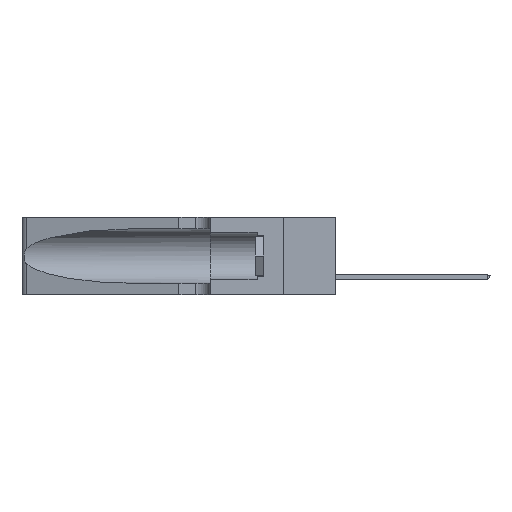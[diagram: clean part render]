
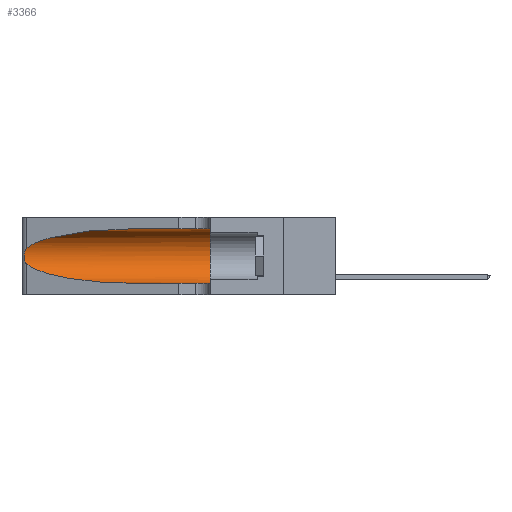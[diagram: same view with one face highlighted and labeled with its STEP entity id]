
A CAD part, left-side view. The second image highlights one B-rep face of the part: STEP entity #3366.
In plain terms, the highlighted cylindrical face has radius 3.308 mm (diameter 6.617 mm), a partial arc.
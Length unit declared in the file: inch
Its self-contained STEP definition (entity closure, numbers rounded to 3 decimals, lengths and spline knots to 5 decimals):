
#304 = CARTESIAN_POINT ( 'NONE',  ( 0.25487, 1.22718, 0.22369 ) ) ;
#501 = CARTESIAN_POINT ( 'NONE',  ( 0.1305, 0.72297, 0.05475 ) ) ;
#1171 = CARTESIAN_POINT ( 'NONE',  ( 0.26017, 1.23833, 0.17102 ) ) ;
#1795 = CARTESIAN_POINT ( 'NONE',  ( 0.1305, 0.35, 0.185 ) ) ;
#1953 = ORIENTED_EDGE ( 'NONE', *, *, #27291, .T. ) ;
#2363 = FACE_OUTER_BOUND ( 'NONE', #25673, .T. ) ;
#2447 = DIRECTION ( 'NONE',  ( 0., -1., 0. ) ) ;
#2669 = VERTEX_POINT ( 'NONE', #20504 ) ;
#2687 = CARTESIAN_POINT ( 'NONE',  ( 0.1305, 0.72297, 0.05475 ) ) ;
#2715 = VERTEX_POINT ( 'NONE', #11101 ) ;
#2776 = CARTESIAN_POINT ( 'NONE',  ( 0.25555, 1.22993, 0.14849 ) ) ;
#3366 = ADVANCED_FACE ( 'NONE', ( #2363 ), #10178, .F. ) ;
#3414 = CARTESIAN_POINT ( 'NONE',  ( 0.25639, 1.23186, 0.15144 ) ) ;
#3592 = LINE ( 'NONE', #9015, #15689 ) ;
#3740 = VERTEX_POINT ( 'NONE', #501 ) ;
#4025 = VERTEX_POINT ( 'NONE', #15299 ) ;
#4188 = EDGE_CURVE ( 'NONE', #17761, #4025, #16731, .T. ) ;
#4283 = CARTESIAN_POINT ( 'NONE',  ( 0.25487, 1.22718, 0.22369 ) ) ;
#4915 = ORIENTED_EDGE ( 'NONE', *, *, #13084, .T. ) ;
#5663 = EDGE_CURVE ( 'NONE', #22052, #2715, #14924, .T. ) ;
#6013 = ORIENTED_EDGE ( 'NONE', *, *, #15741, .T. ) ;
#6236 = DIRECTION ( 'NONE',  ( 0., 1., 0. ) ) ;
#6567 = CARTESIAN_POINT ( 'NONE',  ( 0.1305, 0.72297, 0.31525 ) ) ;
#7114 = CARTESIAN_POINT ( 'NONE',  ( 0.25487, 1.22718, 0.14631 ) ) ;
#9015 = CARTESIAN_POINT ( 'NONE',  ( 0.1305, 1.61858, 0.31525 ) ) ;
#9222 = CARTESIAN_POINT ( 'NONE',  ( 0.1305, 1.61858, 0.185 ) ) ;
#9841 = CARTESIAN_POINT ( 'NONE',  ( 0.25487, 1.22718, 0.22369 ) ) ;
#10178 = CYLINDRICAL_SURFACE ( 'NONE', #22697, 0.13025 ) ;
#11101 = CARTESIAN_POINT ( 'NONE',  ( 0.1305, 0.35, 0.05475 ) ) ;
#11452 =( BOUNDED_CURVE ( )  B_SPLINE_CURVE ( 3, ( #7114, #23000, #16283, #2687 ),
 .UNSPECIFIED., .F., .T. ) 
 B_SPLINE_CURVE_WITH_KNOTS ( ( 4, 4 ),
 ( 3.44316, 4.71239 ),
 .UNSPECIFIED. ) 
 CURVE ( )  GEOMETRIC_REPRESENTATION_ITEM ( )  RATIONAL_B_SPLINE_CURVE ( ( 1., 0.87, 0.87, 1. ) ) 
 REPRESENTATION_ITEM ( '' )  );
#11484 = ORIENTED_EDGE ( 'NONE', *, *, #4188, .T. ) ;
#11900 = CARTESIAN_POINT ( 'NONE',  ( 0.25854, 1.2359, 0.20912 ) ) ;
#12970 = ORIENTED_EDGE ( 'NONE', *, *, #5663, .F. ) ;
#13084 = EDGE_CURVE ( 'NONE', #2669, #17761, #27197, .T. ) ;
#14743 = CARTESIAN_POINT ( 'NONE',  ( 0.26075, 1.23896, 0.178 ) ) ;
#14924 = CIRCLE ( 'NONE', #28054, 0.13025 ) ;
#14928 = ORIENTED_EDGE ( 'NONE', *, *, #18840, .F. ) ;
#15299 = CARTESIAN_POINT ( 'NONE',  ( 0.25487, 1.22718, 0.14631 ) ) ;
#15689 = VECTOR ( 'NONE', #24651, 39.37008 ) ;
#15741 = EDGE_CURVE ( 'NONE', #4025, #3740, #11452, .T. ) ;
#15888 = DIRECTION ( 'NONE',  ( 0., 0., -1. ) ) ;
#16283 = CARTESIAN_POINT ( 'NONE',  ( 0.18966, 0.96281, 0.05475 ) ) ;
#16373 = CARTESIAN_POINT ( 'NONE',  ( 0.25789, 1.23486, 0.15765 ) ) ;
#16461 = CARTESIAN_POINT ( 'NONE',  ( 0.26018, 1.23835, 0.19895 ) ) ;
#16731 = B_SPLINE_CURVE_WITH_KNOTS ( 'NONE', 3,
 ( #304, #18436, #28000, #19046, #11900, #16461, #25520, #14743, #1171, #17009, #16373, #3414, #2776, #20946 ),
 .UNSPECIFIED., .F., .F.,
 ( 4, 2, 2, 2, 2, 2, 4 ),
 ( 0., 0.00027, 0.00053, 0.00107, 0.0016, 0.00187, 0.00214 ),
 .UNSPECIFIED. ) ;
#17009 = CARTESIAN_POINT ( 'NONE',  ( 0.25856, 1.23593, 0.16098 ) ) ;
#17761 = VERTEX_POINT ( 'NONE', #9841 ) ;
#18436 = CARTESIAN_POINT ( 'NONE',  ( 0.25555, 1.22994, 0.2215 ) ) ;
#18607 = CARTESIAN_POINT ( 'NONE',  ( 0.1305, 1.61858, 0.05475 ) ) ;
#18840 = EDGE_CURVE ( 'NONE', #2669, #22052, #3592, .T. ) ;
#19046 = CARTESIAN_POINT ( 'NONE',  ( 0.25787, 1.23484, 0.2124 ) ) ;
#20333 = CARTESIAN_POINT ( 'NONE',  ( 0.1305, 0.35, 0.31525 ) ) ;
#20504 = CARTESIAN_POINT ( 'NONE',  ( 0.1305, 0.72297, 0.31525 ) ) ;
#20729 = DIRECTION ( 'NONE',  ( 0., -1., 0. ) ) ;
#20922 = VECTOR ( 'NONE', #2447, 39.37008 ) ;
#20946 = CARTESIAN_POINT ( 'NONE',  ( 0.25487, 1.22718, 0.14631 ) ) ;
#22052 = VERTEX_POINT ( 'NONE', #20333 ) ;
#22697 = AXIS2_PLACEMENT_3D ( 'NONE', #9222, #20729, #15888 ) ;
#23000 = CARTESIAN_POINT ( 'NONE',  ( 0.2373, 1.15595, 0.08982 ) ) ;
#23101 = CARTESIAN_POINT ( 'NONE',  ( 0.18966, 0.96281, 0.31525 ) ) ;
#23205 = CARTESIAN_POINT ( 'NONE',  ( 0.2373, 1.15595, 0.28018 ) ) ;
#24651 = DIRECTION ( 'NONE',  ( 0., -1., 0. ) ) ;
#25520 = CARTESIAN_POINT ( 'NONE',  ( 0.26075, 1.23896, 0.19203 ) ) ;
#25673 = EDGE_LOOP ( 'NONE', ( #4915, #11484, #6013, #1953, #12970, #14928 ) ) ;
#26425 = DIRECTION ( 'NONE',  ( 0., 0., 1. ) ) ;
#26912 = LINE ( 'NONE', #18607, #20922 ) ;
#27197 =( BOUNDED_CURVE ( )  B_SPLINE_CURVE ( 3, ( #6567, #23101, #23205, #4283 ),
 .UNSPECIFIED., .F., .T. ) 
 B_SPLINE_CURVE_WITH_KNOTS ( ( 4, 4 ),
 ( 1.5708, 2.84003 ),
 .UNSPECIFIED. ) 
 CURVE ( )  GEOMETRIC_REPRESENTATION_ITEM ( )  RATIONAL_B_SPLINE_CURVE ( ( 1., 0.87, 0.87, 1. ) ) 
 REPRESENTATION_ITEM ( '' )  );
#27291 = EDGE_CURVE ( 'NONE', #3740, #2715, #26912, .T. ) ;
#28000 = CARTESIAN_POINT ( 'NONE',  ( 0.25639, 1.23184, 0.21858 ) ) ;
#28054 = AXIS2_PLACEMENT_3D ( 'NONE', #1795, #6236, #26425 ) ;
